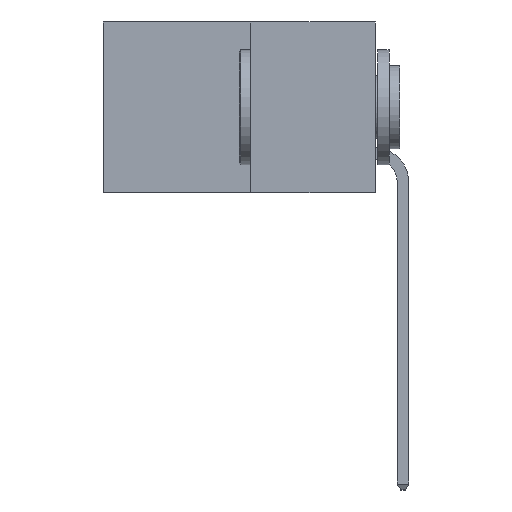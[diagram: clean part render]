
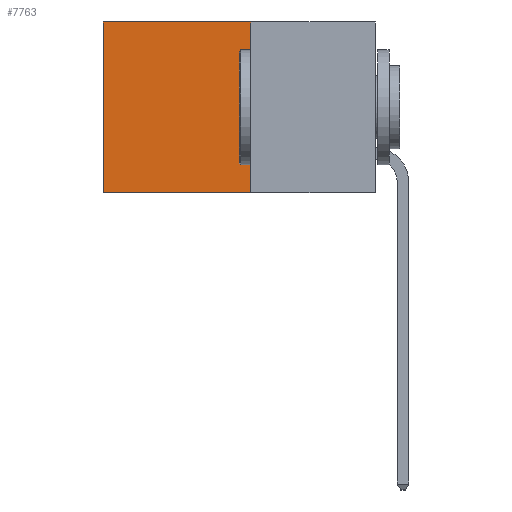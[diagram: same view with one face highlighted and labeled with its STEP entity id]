
A CAD part, left-side view. The second image highlights one B-rep face of the part: STEP entity #7763.
In plain terms, the highlighted planar face has unit normal (-1, 0, 0).
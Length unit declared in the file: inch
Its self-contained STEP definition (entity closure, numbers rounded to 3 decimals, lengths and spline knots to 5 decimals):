
#68 = EDGE_CURVE ( 'NONE', #2087, #3118, #8957, .T. ) ;
#760 = CARTESIAN_POINT ( 'NONE',  ( 0.277, 0.27, -0.37 ) ) ;
#1282 = VECTOR ( 'NONE', #6860, 39.37008 ) ;
#1723 = ORIENTED_EDGE ( 'NONE', *, *, #3965, .F. ) ;
#1818 = LINE ( 'NONE', #5147, #5672 ) ;
#2087 = VERTEX_POINT ( 'NONE', #2283 ) ;
#2132 = VECTOR ( 'NONE', #9593, 39.37008 ) ;
#2283 = CARTESIAN_POINT ( 'NONE',  ( 0.277, 0.27, 0. ) ) ;
#2551 = EDGE_CURVE ( 'NONE', #3118, #3618, #6236, .T. ) ;
#2606 = EDGE_LOOP ( 'NONE', ( #2678, #8375, #1723, #3911 ) ) ;
#2678 = ORIENTED_EDGE ( 'NONE', *, *, #2551, .T. ) ;
#3118 = VERTEX_POINT ( 'NONE', #7656 ) ;
#3618 = VERTEX_POINT ( 'NONE', #8503 ) ;
#3676 = VECTOR ( 'NONE', #9899, 39.37008 ) ;
#3911 = ORIENTED_EDGE ( 'NONE', *, *, #68, .T. ) ;
#3965 = EDGE_CURVE ( 'NONE', #2087, #7221, #9690, .T. ) ;
#4347 = AXIS2_PLACEMENT_3D ( 'NONE', #5821, #5505, #5485 ) ;
#5147 = CARTESIAN_POINT ( 'NONE',  ( 0.277, 0.27, -0.37 ) ) ;
#5346 = DIRECTION ( 'NONE',  ( 0., 1., 0. ) ) ;
#5485 = DIRECTION ( 'NONE',  ( 0., 0., -1. ) ) ;
#5505 = DIRECTION ( 'NONE',  ( 1., 0., 0. ) ) ;
#5640 = EDGE_CURVE ( 'NONE', #7221, #3618, #1818, .T. ) ;
#5651 = PLANE ( 'NONE',  #4347 ) ;
#5672 = VECTOR ( 'NONE', #5346, 39.37008 ) ;
#5821 = CARTESIAN_POINT ( 'NONE',  ( 0.277, 0.27, -0.37 ) ) ;
#6236 = LINE ( 'NONE', #9478, #2132 ) ;
#6860 = DIRECTION ( 'NONE',  ( 0., 1., 0. ) ) ;
#6972 = FACE_OUTER_BOUND ( 'NONE', #2606, .T. ) ;
#7221 = VERTEX_POINT ( 'NONE', #8686 ) ;
#7293 = CARTESIAN_POINT ( 'NONE',  ( 0.277, 0.27, 0. ) ) ;
#7656 = CARTESIAN_POINT ( 'NONE',  ( 0.277, 0.59, 0. ) ) ;
#7763 = ADVANCED_FACE ( 'NONE', ( #6972 ), #5651, .F. ) ;
#8375 = ORIENTED_EDGE ( 'NONE', *, *, #5640, .F. ) ;
#8503 = CARTESIAN_POINT ( 'NONE',  ( 0.277, 0.59, -0.37 ) ) ;
#8686 = CARTESIAN_POINT ( 'NONE',  ( 0.277, 0.27, -0.37 ) ) ;
#8957 = LINE ( 'NONE', #7293, #1282 ) ;
#9478 = CARTESIAN_POINT ( 'NONE',  ( 0.277, 0.59, -0.37 ) ) ;
#9593 = DIRECTION ( 'NONE',  ( 0., 0., -1. ) ) ;
#9690 = LINE ( 'NONE', #760, #3676 ) ;
#9899 = DIRECTION ( 'NONE',  ( 0., 0., -1. ) ) ;
